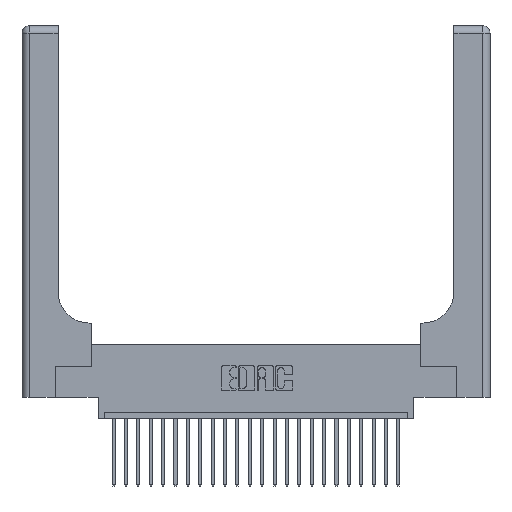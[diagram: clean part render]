
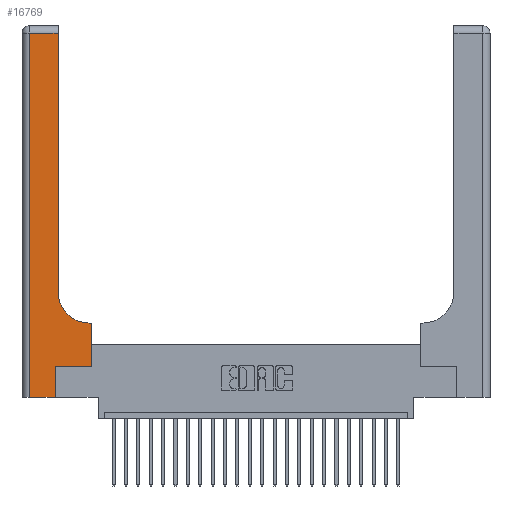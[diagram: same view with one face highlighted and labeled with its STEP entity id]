
A CAD part, top view. The second image highlights one B-rep face of the part: STEP entity #16769.
In plain terms, the highlighted planar face has unit normal (0, 0, 1).
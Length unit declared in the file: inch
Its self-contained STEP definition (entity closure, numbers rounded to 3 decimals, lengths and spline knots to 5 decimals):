
#388 = CARTESIAN_POINT ( 'NONE',  ( 0.5415, 0.6, 0.37 ) ) ;
#442 = DIRECTION ( 'NONE',  ( 0., -1., 0. ) ) ;
#939 = ORIENTED_EDGE ( 'NONE', *, *, #21638, .T. ) ;
#1049 = CARTESIAN_POINT ( 'NONE',  ( 0., 3., 0.37 ) ) ;
#1533 = FACE_OUTER_BOUND ( 'NONE', #18080, .T. ) ;
#1799 = ORIENTED_EDGE ( 'NONE', *, *, #5165, .T. ) ;
#1974 = VECTOR ( 'NONE', #13137, 39.37008 ) ;
#2083 = CARTESIAN_POINT ( 'NONE',  ( 0.5585, 0.25, 0.37 ) ) ;
#2089 = VERTEX_POINT ( 'NONE', #19325 ) ;
#2310 = CARTESIAN_POINT ( 'NONE',  ( 0.2915, 0.6, 0.37 ) ) ;
#2432 = DIRECTION ( 'NONE',  ( 0., 0., -1. ) ) ;
#3270 = LINE ( 'NONE', #13060, #18201 ) ;
#3305 = CARTESIAN_POINT ( 'NONE',  ( 0.269, 0., 0.37 ) ) ;
#3815 = DIRECTION ( 'NONE',  ( 0., 1., 0. ) ) ;
#3889 = VERTEX_POINT ( 'NONE', #388 ) ;
#4230 = EDGE_CURVE ( 'NONE', #19980, #3889, #7641, .T. ) ;
#4814 = PLANE ( 'NONE',  #7694 ) ;
#5165 = EDGE_CURVE ( 'NONE', #3889, #18558, #20651, .T. ) ;
#6098 = DIRECTION ( 'NONE',  ( 1., 0., 0. ) ) ;
#6660 = DIRECTION ( 'NONE',  ( 0., 0., -1. ) ) ;
#6722 = CARTESIAN_POINT ( 'NONE',  ( 0.269, 0.25, 0.37 ) ) ;
#7047 = ORIENTED_EDGE ( 'NONE', *, *, #24474, .T. ) ;
#7094 = CARTESIAN_POINT ( 'NONE',  ( 0., 2.94, 0.37 ) ) ;
#7353 = LINE ( 'NONE', #7094, #19808 ) ;
#7546 = VERTEX_POINT ( 'NONE', #16160 ) ;
#7641 = LINE ( 'NONE', #2310, #20692 ) ;
#7694 = AXIS2_PLACEMENT_3D ( 'NONE', #1049, #6660, #9002 ) ;
#8093 = CARTESIAN_POINT ( 'NONE',  ( 0.5415, 0.85, 0.37 ) ) ;
#9002 = DIRECTION ( 'NONE',  ( -1., 0., 0. ) ) ;
#9898 = LINE ( 'NONE', #3305, #22972 ) ;
#9930 = ORIENTED_EDGE ( 'NONE', *, *, #23932, .T. ) ;
#10368 = CARTESIAN_POINT ( 'NONE',  ( 0.06, 3., 0.37 ) ) ;
#10781 = CARTESIAN_POINT ( 'NONE',  ( 0.06, 2.94, 0.37 ) ) ;
#11341 = CARTESIAN_POINT ( 'NONE',  ( 0., 0., 0.37 ) ) ;
#11793 = EDGE_CURVE ( 'NONE', #17058, #21782, #15641, .T. ) ;
#12718 = CARTESIAN_POINT ( 'NONE',  ( 0.5585, 0.6, 0.37 ) ) ;
#12861 = VECTOR ( 'NONE', #14465, 39.37008 ) ;
#13060 = CARTESIAN_POINT ( 'NONE',  ( 0.2915, 3., 0.37 ) ) ;
#13137 = DIRECTION ( 'NONE',  ( 1., 0., 0. ) ) ;
#14272 = LINE ( 'NONE', #10368, #19573 ) ;
#14430 = LINE ( 'NONE', #11341, #1974 ) ;
#14465 = DIRECTION ( 'NONE',  ( 1., 0., 0. ) ) ;
#14539 = CARTESIAN_POINT ( 'NONE',  ( 0.5585, 0.25, 0.37 ) ) ;
#14632 = EDGE_CURVE ( 'NONE', #20352, #7546, #14430, .T. ) ;
#15641 = LINE ( 'NONE', #6722, #12861 ) ;
#15781 = EDGE_CURVE ( 'NONE', #21782, #19980, #22496, .T. ) ;
#16160 = CARTESIAN_POINT ( 'NONE',  ( 0.269, 0., 0.37 ) ) ;
#16769 = ADVANCED_FACE ( 'NONE', ( #1533 ), #4814, .F. ) ;
#17058 = VERTEX_POINT ( 'NONE', #17130 ) ;
#17130 = CARTESIAN_POINT ( 'NONE',  ( 0.269, 0.25, 0.37 ) ) ;
#17280 = CARTESIAN_POINT ( 'NONE',  ( 0.2915, 0.85, 0.37 ) ) ;
#18080 = EDGE_LOOP ( 'NONE', ( #7047, #9930, #939, #20324, #20632, #21376, #25810, #23762, #1799 ) ) ;
#18201 = VECTOR ( 'NONE', #25094, 39.37008 ) ;
#18360 = EDGE_CURVE ( 'NONE', #7546, #17058, #9898, .T. ) ;
#18558 = VERTEX_POINT ( 'NONE', #17280 ) ;
#19325 = CARTESIAN_POINT ( 'NONE',  ( 0.2915, 2.94, 0.37 ) ) ;
#19544 = DIRECTION ( 'NONE',  ( -1., 0., 0. ) ) ;
#19573 = VECTOR ( 'NONE', #442, 39.37008 ) ;
#19808 = VECTOR ( 'NONE', #19544, 39.37008 ) ;
#19978 = VECTOR ( 'NONE', #3815, 39.37008 ) ;
#19980 = VERTEX_POINT ( 'NONE', #12718 ) ;
#20324 = ORIENTED_EDGE ( 'NONE', *, *, #14632, .T. ) ;
#20352 = VERTEX_POINT ( 'NONE', #22029 ) ;
#20632 = ORIENTED_EDGE ( 'NONE', *, *, #18360, .T. ) ;
#20651 = CIRCLE ( 'NONE', #21034, 0.25 ) ;
#20692 = VECTOR ( 'NONE', #24375, 39.37008 ) ;
#20984 = DIRECTION ( 'NONE',  ( 0., 1., 0. ) ) ;
#21034 = AXIS2_PLACEMENT_3D ( 'NONE', #8093, #2432, #6098 ) ;
#21376 = ORIENTED_EDGE ( 'NONE', *, *, #11793, .T. ) ;
#21638 = EDGE_CURVE ( 'NONE', #22479, #20352, #14272, .T. ) ;
#21782 = VERTEX_POINT ( 'NONE', #14539 ) ;
#22029 = CARTESIAN_POINT ( 'NONE',  ( 0.06, 0., 0.37 ) ) ;
#22479 = VERTEX_POINT ( 'NONE', #10781 ) ;
#22496 = LINE ( 'NONE', #2083, #19978 ) ;
#22972 = VECTOR ( 'NONE', #20984, 39.37008 ) ;
#23762 = ORIENTED_EDGE ( 'NONE', *, *, #4230, .T. ) ;
#23932 = EDGE_CURVE ( 'NONE', #2089, #22479, #7353, .T. ) ;
#24375 = DIRECTION ( 'NONE',  ( -1., 0., 0. ) ) ;
#24474 = EDGE_CURVE ( 'NONE', #18558, #2089, #3270, .T. ) ;
#25094 = DIRECTION ( 'NONE',  ( 0., 1., 0. ) ) ;
#25810 = ORIENTED_EDGE ( 'NONE', *, *, #15781, .T. ) ;
